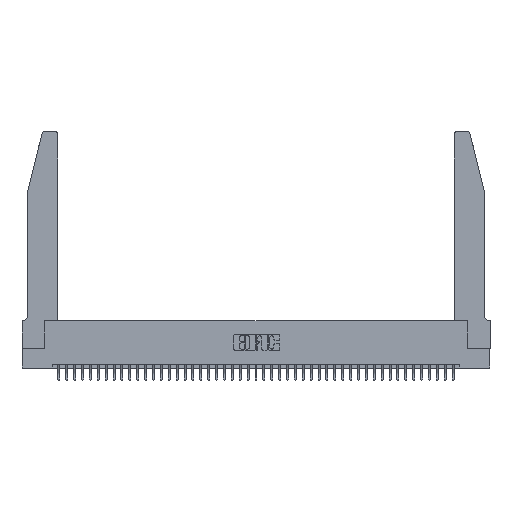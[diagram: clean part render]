
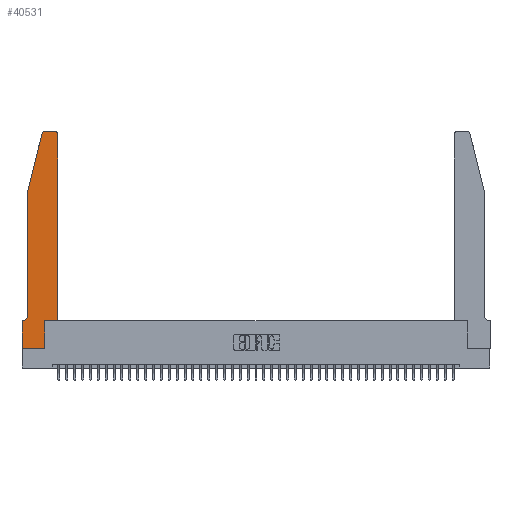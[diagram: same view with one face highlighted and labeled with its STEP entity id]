
A CAD part, top view. The second image highlights one B-rep face of the part: STEP entity #40531.
In plain terms, the highlighted planar face has unit normal (0, 0, 1).
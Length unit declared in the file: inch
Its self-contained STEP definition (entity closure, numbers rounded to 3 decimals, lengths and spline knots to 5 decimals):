
#569 = LINE ( 'NONE', #15594, #9807 ) ;
#1411 = ORIENTED_EDGE ( 'NONE', *, *, #10852, .T. ) ;
#1511 = ORIENTED_EDGE ( 'NONE', *, *, #26394, .T. ) ;
#1775 = CARTESIAN_POINT ( 'NONE',  ( 0.0055, 0.35, 0.37 ) ) ;
#2224 = CARTESIAN_POINT ( 'NONE',  ( 0.2865, 0., 0.37 ) ) ;
#3305 = VECTOR ( 'NONE', #20057, 39.37008 ) ;
#3824 = EDGE_CURVE ( 'NONE', #33844, #9358, #17164, .T. ) ;
#4340 = ORIENTED_EDGE ( 'NONE', *, *, #32120, .T. ) ;
#4365 = LINE ( 'NONE', #43383, #3305 ) ;
#6574 = CARTESIAN_POINT ( 'NONE',  ( 0.0755, 0.35, 0.37 ) ) ;
#6720 = CARTESIAN_POINT ( 'NONE',  ( 0.4205, 2.75, 0.37 ) ) ;
#7372 = CARTESIAN_POINT ( 'NONE',  ( 0., 0., 0.37 ) ) ;
#7599 = EDGE_CURVE ( 'NONE', #41041, #19039, #39951, .T. ) ;
#8175 = EDGE_LOOP ( 'NONE', ( #1411, #24628, #30367, #22808, #33806, #15482, #43584, #20102, #39347, #38283, #1511, #4340 ) ) ;
#8678 = CIRCLE ( 'NONE', #33191, 0.07 ) ;
#8916 = CARTESIAN_POINT ( 'NONE',  ( 0.4505, 2.72, 0.37 ) ) ;
#9215 = DIRECTION ( 'NONE',  ( 0., 0., 1. ) ) ;
#9358 = VERTEX_POINT ( 'NONE', #19702 ) ;
#9395 = EDGE_CURVE ( 'NONE', #19268, #41534, #25273, .T. ) ;
#9807 = VECTOR ( 'NONE', #32260, 39.37008 ) ;
#10693 = DIRECTION ( 'NONE',  ( 0., 0., 1. ) ) ;
#10852 = EDGE_CURVE ( 'NONE', #24541, #19268, #569, .T. ) ;
#11499 = CARTESIAN_POINT ( 'NONE',  ( 0.4505, 0.35, 0.37 ) ) ;
#12052 = LINE ( 'NONE', #13709, #36639 ) ;
#13385 = CARTESIAN_POINT ( 'NONE',  ( 0.284, 2.72, 0.37 ) ) ;
#13709 = CARTESIAN_POINT ( 'NONE',  ( 0., 0., 0.37 ) ) ;
#14184 = LINE ( 'NONE', #18265, #31949 ) ;
#14686 = AXIS2_PLACEMENT_3D ( 'NONE', #29468, #9215, #32793 ) ;
#15004 = CARTESIAN_POINT ( 'NONE',  ( 0.0055, 0.42, 0.37 ) ) ;
#15482 = ORIENTED_EDGE ( 'NONE', *, *, #32677, .T. ) ;
#15527 = FACE_OUTER_BOUND ( 'NONE', #8175, .T. ) ;
#15594 = CARTESIAN_POINT ( 'NONE',  ( 0.2605, 2.75, 0.37 ) ) ;
#15807 = CARTESIAN_POINT ( 'NONE',  ( 0., 0.35, 0.37 ) ) ;
#15983 = CARTESIAN_POINT ( 'NONE',  ( 0.4505, 0.35, 0.37 ) ) ;
#16748 = DIRECTION ( 'NONE',  ( 1., 0., 0. ) ) ;
#17164 = LINE ( 'NONE', #7372, #33892 ) ;
#17208 = LINE ( 'NONE', #22260, #26181 ) ;
#17717 = CARTESIAN_POINT ( 'NONE',  ( 0.0755, 0.42, 0.37 ) ) ;
#18265 = CARTESIAN_POINT ( 'NONE',  ( 0.0755, 2., 0.37 ) ) ;
#18385 = DIRECTION ( 'NONE',  ( -1., 0., 0. ) ) ;
#19039 = VERTEX_POINT ( 'NONE', #17717 ) ;
#19268 = VERTEX_POINT ( 'NONE', #43011 ) ;
#19384 = AXIS2_PLACEMENT_3D ( 'NONE', #13385, #36731, #16748 ) ;
#19544 = CIRCLE ( 'NONE', #25196, 0.03 ) ;
#19702 = CARTESIAN_POINT ( 'NONE',  ( 0., 0., 0.37 ) ) ;
#20057 = DIRECTION ( 'NONE',  ( 0., 1., 0. ) ) ;
#20102 = ORIENTED_EDGE ( 'NONE', *, *, #24564, .T. ) ;
#22260 = CARTESIAN_POINT ( 'NONE',  ( 0.4505, 0.35, 0.37 ) ) ;
#22808 = ORIENTED_EDGE ( 'NONE', *, *, #7599, .T. ) ;
#23188 = VECTOR ( 'NONE', #36894, 39.37008 ) ;
#24541 = VERTEX_POINT ( 'NONE', #6720 ) ;
#24564 = EDGE_CURVE ( 'NONE', #9358, #28289, #12052, .T. ) ;
#24628 = ORIENTED_EDGE ( 'NONE', *, *, #9395, .T. ) ;
#25196 = AXIS2_PLACEMENT_3D ( 'NONE', #30858, #10693, #34185 ) ;
#25273 = CIRCLE ( 'NONE', #19384, 0.03 ) ;
#25631 = DIRECTION ( 'NONE',  ( 1., 0., 0. ) ) ;
#26181 = VECTOR ( 'NONE', #25631, 39.37008 ) ;
#26301 = VERTEX_POINT ( 'NONE', #1775 ) ;
#26394 = EDGE_CURVE ( 'NONE', #33638, #30566, #31698, .T. ) ;
#27827 = DIRECTION ( 'NONE',  ( 0., -1., 0. ) ) ;
#28289 = VERTEX_POINT ( 'NONE', #2224 ) ;
#28348 = DIRECTION ( 'NONE',  ( 0., -1., 0. ) ) ;
#29263 = EDGE_CURVE ( 'NONE', #41534, #41041, #14184, .T. ) ;
#29468 = CARTESIAN_POINT ( 'NONE',  ( 0., 0.35, 0.37 ) ) ;
#29526 = EDGE_CURVE ( 'NONE', #28289, #42514, #4365, .T. ) ;
#29837 = EDGE_CURVE ( 'NONE', #19039, #26301, #8678, .T. ) ;
#30367 = ORIENTED_EDGE ( 'NONE', *, *, #29263, .T. ) ;
#30566 = VERTEX_POINT ( 'NONE', #8916 ) ;
#30858 = CARTESIAN_POINT ( 'NONE',  ( 0.4205, 2.72, 0.37 ) ) ;
#31123 = VECTOR ( 'NONE', #28348, 39.37008 ) ;
#31698 = LINE ( 'NONE', #15983, #39484 ) ;
#31949 = VECTOR ( 'NONE', #41609, 39.37008 ) ;
#32120 = EDGE_CURVE ( 'NONE', #30566, #24541, #19544, .T. ) ;
#32166 = CARTESIAN_POINT ( 'NONE',  ( 0.0755, 2., 0.37 ) ) ;
#32260 = DIRECTION ( 'NONE',  ( -1., 0., 0. ) ) ;
#32677 = EDGE_CURVE ( 'NONE', #26301, #33844, #33069, .T. ) ;
#32793 = DIRECTION ( 'NONE',  ( 1., 0., 0. ) ) ;
#33069 = LINE ( 'NONE', #6574, #23188 ) ;
#33191 = AXIS2_PLACEMENT_3D ( 'NONE', #15004, #38359, #18385 ) ;
#33638 = VERTEX_POINT ( 'NONE', #11499 ) ;
#33705 = DIRECTION ( 'NONE',  ( 1., 0., 0. ) ) ;
#33806 = ORIENTED_EDGE ( 'NONE', *, *, #29837, .T. ) ;
#33844 = VERTEX_POINT ( 'NONE', #15807 ) ;
#33892 = VECTOR ( 'NONE', #27827, 39.37008 ) ;
#34185 = DIRECTION ( 'NONE',  ( 1., 0., 0. ) ) ;
#34375 = EDGE_CURVE ( 'NONE', #42514, #33638, #17208, .T. ) ;
#36639 = VECTOR ( 'NONE', #33705, 39.37008 ) ;
#36706 = CARTESIAN_POINT ( 'NONE',  ( 0.2865, 0.35, 0.37 ) ) ;
#36731 = DIRECTION ( 'NONE',  ( 0., 0., 1. ) ) ;
#36894 = DIRECTION ( 'NONE',  ( -1., 0., 0. ) ) ;
#38283 = ORIENTED_EDGE ( 'NONE', *, *, #34375, .T. ) ;
#38359 = DIRECTION ( 'NONE',  ( 0., 0., -1. ) ) ;
#39347 = ORIENTED_EDGE ( 'NONE', *, *, #29526, .T. ) ;
#39455 = DIRECTION ( 'NONE',  ( 0., 1., 0. ) ) ;
#39484 = VECTOR ( 'NONE', #39455, 39.37008 ) ;
#39951 = LINE ( 'NONE', #41566, #31123 ) ;
#40531 = ADVANCED_FACE ( 'NONE', ( #15527 ), #42723, .T. ) ;
#41003 = CARTESIAN_POINT ( 'NONE',  ( 0.25487, 2.72718, 0.37 ) ) ;
#41041 = VERTEX_POINT ( 'NONE', #32166 ) ;
#41534 = VERTEX_POINT ( 'NONE', #41003 ) ;
#41566 = CARTESIAN_POINT ( 'NONE',  ( 0.0755, 2., 0.37 ) ) ;
#41609 = DIRECTION ( 'NONE',  ( -0.239, -0.971, 0. ) ) ;
#42514 = VERTEX_POINT ( 'NONE', #36706 ) ;
#42723 = PLANE ( 'NONE',  #14686 ) ;
#43011 = CARTESIAN_POINT ( 'NONE',  ( 0.284, 2.75, 0.37 ) ) ;
#43383 = CARTESIAN_POINT ( 'NONE',  ( 0.2865, 0.35, 0.37 ) ) ;
#43584 = ORIENTED_EDGE ( 'NONE', *, *, #3824, .T. ) ;
